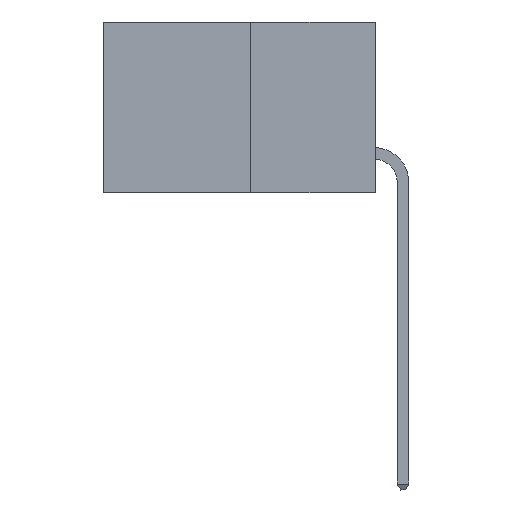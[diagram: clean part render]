
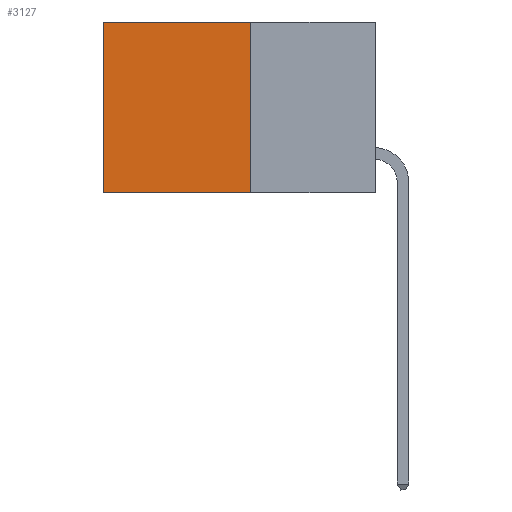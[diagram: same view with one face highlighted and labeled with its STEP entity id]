
A CAD part, left-side view. The second image highlights one B-rep face of the part: STEP entity #3127.
In plain terms, the highlighted planar face has unit normal (-1, 0, 0).
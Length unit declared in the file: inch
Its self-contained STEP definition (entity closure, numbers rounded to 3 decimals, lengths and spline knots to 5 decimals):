
#699 = VERTEX_POINT ( 'NONE', #8479 ) ;
#902 = CARTESIAN_POINT ( 'NONE',  ( 0.277, 0.27, -0.37 ) ) ;
#1128 = VECTOR ( 'NONE', #2452, 39.37008 ) ;
#1275 = EDGE_CURVE ( 'NONE', #7307, #6286, #6550, .T. ) ;
#1567 = EDGE_CURVE ( 'NONE', #6286, #699, #2520, .T. ) ;
#1929 = ORIENTED_EDGE ( 'NONE', *, *, #1567, .F. ) ;
#2452 = DIRECTION ( 'NONE',  ( 0., 1., 0. ) ) ;
#2520 = LINE ( 'NONE', #7907, #7577 ) ;
#2592 = CARTESIAN_POINT ( 'NONE',  ( 0.277, 0.27, -0.37 ) ) ;
#3063 = VECTOR ( 'NONE', #3315, 39.37008 ) ;
#3127 = ADVANCED_FACE ( 'NONE', ( #5193 ), #3776, .F. ) ;
#3315 = DIRECTION ( 'NONE',  ( 0., 0., -1. ) ) ;
#3719 = ORIENTED_EDGE ( 'NONE', *, *, #5414, .T. ) ;
#3730 = EDGE_CURVE ( 'NONE', #7307, #7846, #5994, .T. ) ;
#3776 = PLANE ( 'NONE',  #5552 ) ;
#3817 = DIRECTION ( 'NONE',  ( 0., 1., 0. ) ) ;
#3888 = CARTESIAN_POINT ( 'NONE',  ( 0.277, 0.59, 0. ) ) ;
#3945 = CARTESIAN_POINT ( 'NONE',  ( 0.277, 0.59, -0.37 ) ) ;
#4110 = ORIENTED_EDGE ( 'NONE', *, *, #3730, .T. ) ;
#4316 = ORIENTED_EDGE ( 'NONE', *, *, #1275, .F. ) ;
#4364 = CARTESIAN_POINT ( 'NONE',  ( 0.277, 0.27, -0.37 ) ) ;
#4488 = CARTESIAN_POINT ( 'NONE',  ( 0.277, 0.27, 0. ) ) ;
#4841 = VECTOR ( 'NONE', #6763, 39.37008 ) ;
#5076 = EDGE_LOOP ( 'NONE', ( #3719, #1929, #4316, #4110 ) ) ;
#5193 = FACE_OUTER_BOUND ( 'NONE', #5076, .T. ) ;
#5414 = EDGE_CURVE ( 'NONE', #7846, #699, #7190, .T. ) ;
#5552 = AXIS2_PLACEMENT_3D ( 'NONE', #2592, #8285, #8322 ) ;
#5994 = LINE ( 'NONE', #4488, #1128 ) ;
#6286 = VERTEX_POINT ( 'NONE', #902 ) ;
#6550 = LINE ( 'NONE', #4364, #4841 ) ;
#6763 = DIRECTION ( 'NONE',  ( 0., 0., -1. ) ) ;
#7190 = LINE ( 'NONE', #3945, #3063 ) ;
#7307 = VERTEX_POINT ( 'NONE', #7941 ) ;
#7577 = VECTOR ( 'NONE', #3817, 39.37008 ) ;
#7846 = VERTEX_POINT ( 'NONE', #3888 ) ;
#7907 = CARTESIAN_POINT ( 'NONE',  ( 0.277, 0.27, -0.37 ) ) ;
#7941 = CARTESIAN_POINT ( 'NONE',  ( 0.277, 0.27, 0. ) ) ;
#8285 = DIRECTION ( 'NONE',  ( 1., 0., 0. ) ) ;
#8322 = DIRECTION ( 'NONE',  ( 0., 0., -1. ) ) ;
#8479 = CARTESIAN_POINT ( 'NONE',  ( 0.277, 0.59, -0.37 ) ) ;
